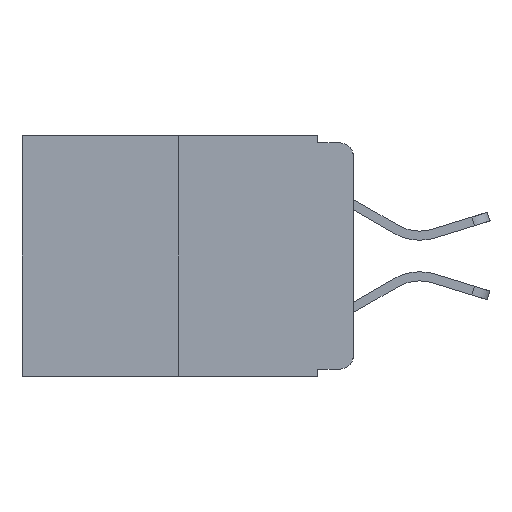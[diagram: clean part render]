
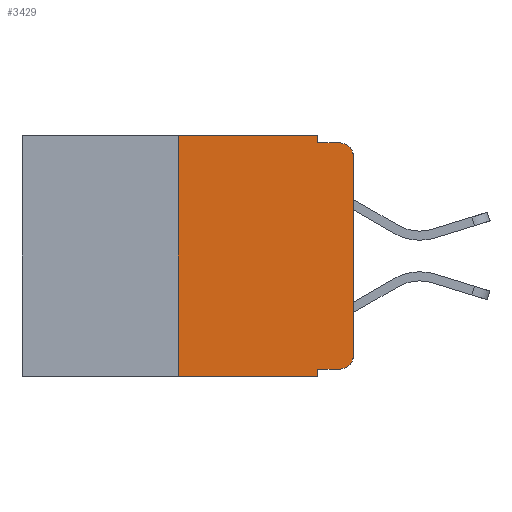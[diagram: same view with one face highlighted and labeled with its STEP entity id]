
A CAD part, left-side view. The second image highlights one B-rep face of the part: STEP entity #3429.
In plain terms, the highlighted planar face has unit normal (-1, 0, 0).
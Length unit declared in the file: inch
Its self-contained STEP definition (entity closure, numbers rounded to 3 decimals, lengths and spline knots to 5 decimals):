
#259 = EDGE_CURVE ( 'NONE', #1268, #13861, #6541, .T. ) ;
#380 = VERTEX_POINT ( 'NONE', #1183 ) ;
#530 = CIRCLE ( 'NONE', #10360, 0.02 ) ;
#753 = PLANE ( 'NONE',  #3991 ) ;
#974 = DIRECTION ( 'NONE',  ( -1., 0., 0. ) ) ;
#1102 = VERTEX_POINT ( 'NONE', #10908 ) ;
#1167 = EDGE_CURVE ( 'NONE', #1102, #1268, #14007, .T. ) ;
#1183 = CARTESIAN_POINT ( 'NONE',  ( 0., 0.051, -0.01 ) ) ;
#1212 = ORIENTED_EDGE ( 'NONE', *, *, #259, .T. ) ;
#1268 = VERTEX_POINT ( 'NONE', #5938 ) ;
#1309 = LINE ( 'NONE', #15150, #13425 ) ;
#1322 = DIRECTION ( 'NONE',  ( 0., -1., 0. ) ) ;
#2012 = ORIENTED_EDGE ( 'NONE', *, *, #13277, .F. ) ;
#2076 = DIRECTION ( 'NONE',  ( 1., 0., 0. ) ) ;
#2423 = ORIENTED_EDGE ( 'NONE', *, *, #11825, .T. ) ;
#2493 = VECTOR ( 'NONE', #14372, 39.37008 ) ;
#2540 = CARTESIAN_POINT ( 'NONE',  ( 0., 0.02, -0.01 ) ) ;
#2719 = DIRECTION ( 'NONE',  ( 0., -1., 0. ) ) ;
#2858 = LINE ( 'NONE', #13267, #2493 ) ;
#3196 = VERTEX_POINT ( 'NONE', #4649 ) ;
#3429 = ADVANCED_FACE ( 'NONE', ( #6325 ), #753, .F. ) ;
#3670 = DIRECTION ( 'NONE',  ( 0., 0., 1. ) ) ;
#3991 = AXIS2_PLACEMENT_3D ( 'NONE', #11455, #2076, #10326 ) ;
#4068 = CARTESIAN_POINT ( 'NONE',  ( 0., 0.25, 0. ) ) ;
#4254 = CARTESIAN_POINT ( 'NONE',  ( 0., 0.02, -0.03 ) ) ;
#4458 = DIRECTION ( 'NONE',  ( 0., 0., -1. ) ) ;
#4649 = CARTESIAN_POINT ( 'NONE',  ( 0., 0.051, -0.343 ) ) ;
#5013 = VERTEX_POINT ( 'NONE', #7669 ) ;
#5505 = VERTEX_POINT ( 'NONE', #14152 ) ;
#5776 = DIRECTION ( 'NONE',  ( -1., 0., 0. ) ) ;
#5785 = EDGE_CURVE ( 'NONE', #14242, #3196, #11915, .T. ) ;
#5938 = CARTESIAN_POINT ( 'NONE',  ( 0., 0., -0.03 ) ) ;
#5985 = EDGE_CURVE ( 'NONE', #8795, #5505, #6265, .T. ) ;
#6265 = LINE ( 'NONE', #15244, #12091 ) ;
#6325 = FACE_OUTER_BOUND ( 'NONE', #12032, .T. ) ;
#6456 = VECTOR ( 'NONE', #10256, 39.37008 ) ;
#6541 = CIRCLE ( 'NONE', #11373, 0.02 ) ;
#7126 = LINE ( 'NONE', #12038, #12864 ) ;
#7626 = ORIENTED_EDGE ( 'NONE', *, *, #14751, .F. ) ;
#7669 = CARTESIAN_POINT ( 'NONE',  ( 0., 0.051, -0.333 ) ) ;
#7789 = VERTEX_POINT ( 'NONE', #8138 ) ;
#7971 = ORIENTED_EDGE ( 'NONE', *, *, #14012, .F. ) ;
#8138 = CARTESIAN_POINT ( 'NONE',  ( 0., 0.02, -0.333 ) ) ;
#8331 = ORIENTED_EDGE ( 'NONE', *, *, #5785, .T. ) ;
#8623 = LINE ( 'NONE', #11514, #14309 ) ;
#8795 = VERTEX_POINT ( 'NONE', #4068 ) ;
#9094 = CARTESIAN_POINT ( 'NONE',  ( 0., 0.473, -0.343 ) ) ;
#10256 = DIRECTION ( 'NONE',  ( 0., -1., 0. ) ) ;
#10326 = DIRECTION ( 'NONE',  ( 0., 0., -1. ) ) ;
#10360 = AXIS2_PLACEMENT_3D ( 'NONE', #12695, #5776, #13783 ) ;
#10633 = LINE ( 'NONE', #13197, #13291 ) ;
#10908 = CARTESIAN_POINT ( 'NONE',  ( 0., 0., -0.313 ) ) ;
#11026 = EDGE_CURVE ( 'NONE', #7789, #1102, #530, .T. ) ;
#11072 = ORIENTED_EDGE ( 'NONE', *, *, #5985, .F. ) ;
#11373 = AXIS2_PLACEMENT_3D ( 'NONE', #4254, #974, #4458 ) ;
#11455 = CARTESIAN_POINT ( 'NONE',  ( 0., 0.473, 0. ) ) ;
#11514 = CARTESIAN_POINT ( 'NONE',  ( 0., 0.051, 0. ) ) ;
#11825 = EDGE_CURVE ( 'NONE', #5013, #7789, #10633, .T. ) ;
#11915 = LINE ( 'NONE', #9094, #6456 ) ;
#12032 = EDGE_LOOP ( 'NONE', ( #12999, #1212, #7626, #7971, #11072, #2012, #8331, #14378, #2423, #14709 ) ) ;
#12038 = CARTESIAN_POINT ( 'NONE',  ( 0., 0.051, -0.01 ) ) ;
#12085 = DIRECTION ( 'NONE',  ( 0., -1., 0. ) ) ;
#12091 = VECTOR ( 'NONE', #1322, 39.37008 ) ;
#12116 = CARTESIAN_POINT ( 'NONE',  ( 0., 0., 0. ) ) ;
#12569 = CARTESIAN_POINT ( 'NONE',  ( 0., 0.25, -0.343 ) ) ;
#12575 = EDGE_CURVE ( 'NONE', #5013, #3196, #8623, .T. ) ;
#12641 = DIRECTION ( 'NONE',  ( 0., 0., -1. ) ) ;
#12695 = CARTESIAN_POINT ( 'NONE',  ( 0., 0.02, -0.313 ) ) ;
#12864 = VECTOR ( 'NONE', #12085, 39.37008 ) ;
#12999 = ORIENTED_EDGE ( 'NONE', *, *, #1167, .T. ) ;
#13197 = CARTESIAN_POINT ( 'NONE',  ( 0., 0.051, -0.333 ) ) ;
#13267 = CARTESIAN_POINT ( 'NONE',  ( 0., 0.051, 0. ) ) ;
#13277 = EDGE_CURVE ( 'NONE', #14242, #8795, #1309, .T. ) ;
#13291 = VECTOR ( 'NONE', #2719, 39.37008 ) ;
#13323 = VECTOR ( 'NONE', #3670, 39.37008 ) ;
#13425 = VECTOR ( 'NONE', #14103, 39.37008 ) ;
#13783 = DIRECTION ( 'NONE',  ( 0., 0., -1. ) ) ;
#13861 = VERTEX_POINT ( 'NONE', #2540 ) ;
#14007 = LINE ( 'NONE', #12116, #13323 ) ;
#14012 = EDGE_CURVE ( 'NONE', #5505, #380, #2858, .T. ) ;
#14103 = DIRECTION ( 'NONE',  ( 0., 0., 1. ) ) ;
#14152 = CARTESIAN_POINT ( 'NONE',  ( 0., 0.051, 0. ) ) ;
#14242 = VERTEX_POINT ( 'NONE', #12569 ) ;
#14309 = VECTOR ( 'NONE', #12641, 39.37008 ) ;
#14372 = DIRECTION ( 'NONE',  ( 0., 0., -1. ) ) ;
#14378 = ORIENTED_EDGE ( 'NONE', *, *, #12575, .F. ) ;
#14709 = ORIENTED_EDGE ( 'NONE', *, *, #11026, .T. ) ;
#14751 = EDGE_CURVE ( 'NONE', #380, #13861, #7126, .T. ) ;
#15150 = CARTESIAN_POINT ( 'NONE',  ( 0., 0.25, 0. ) ) ;
#15244 = CARTESIAN_POINT ( 'NONE',  ( 0., 0.473, 0. ) ) ;
